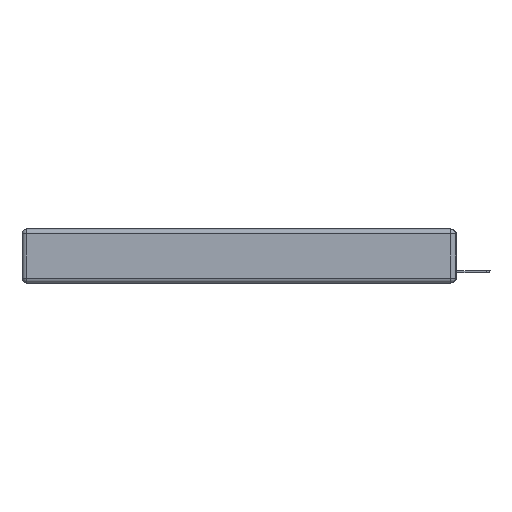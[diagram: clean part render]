
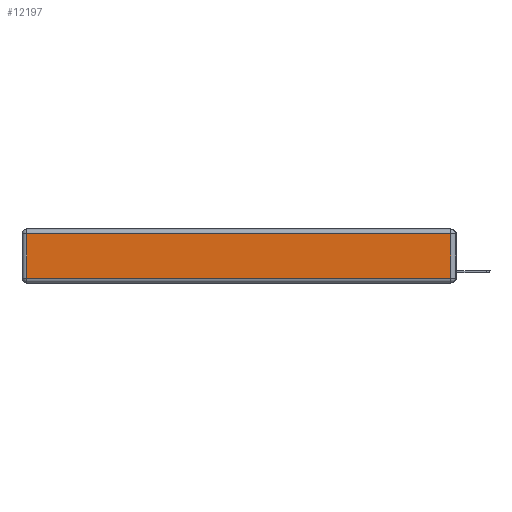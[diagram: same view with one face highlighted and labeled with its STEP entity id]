
A CAD part, left-side view. The second image highlights one B-rep face of the part: STEP entity #12197.
In plain terms, the highlighted planar face has unit normal (-1, 0, 0).
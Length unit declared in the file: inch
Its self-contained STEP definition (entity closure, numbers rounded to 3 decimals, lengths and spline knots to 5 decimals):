
#1809 = AXIS2_PLACEMENT_3D ( 'NONE', #8646, #13525, #8936 ) ;
#2322 = CARTESIAN_POINT ( 'NONE',  ( 0., 0.03, -0.03 ) ) ;
#3725 = EDGE_CURVE ( 'NONE', #6217, #6629, #13853, .T. ) ;
#4419 = ORIENTED_EDGE ( 'NONE', *, *, #15824, .T. ) ;
#4536 = LINE ( 'NONE', #9235, #6363 ) ;
#5135 = PLANE ( 'NONE',  #1809 ) ;
#6217 = VERTEX_POINT ( 'NONE', #11369 ) ;
#6363 = VECTOR ( 'NONE', #21067, 39.37008 ) ;
#6536 = LINE ( 'NONE', #21518, #16589 ) ;
#6629 = VERTEX_POINT ( 'NONE', #2322 ) ;
#7221 = CARTESIAN_POINT ( 'NONE',  ( 0., 2.72, -0.343 ) ) ;
#7976 = DIRECTION ( 'NONE',  ( 0., 0., 1. ) ) ;
#8363 = VERTEX_POINT ( 'NONE', #20079 ) ;
#8646 = CARTESIAN_POINT ( 'NONE',  ( 0., 0., -0.343 ) ) ;
#8843 = DIRECTION ( 'NONE',  ( 0., 0., -1. ) ) ;
#8936 = DIRECTION ( 'NONE',  ( 0., 0., 1. ) ) ;
#9235 = CARTESIAN_POINT ( 'NONE',  ( 0., 2.75, -0.03 ) ) ;
#9616 = VECTOR ( 'NONE', #8843, 39.37008 ) ;
#9675 = EDGE_CURVE ( 'NONE', #6629, #8363, #4536, .T. ) ;
#10180 = EDGE_CURVE ( 'NONE', #8363, #13931, #19923, .T. ) ;
#11369 = CARTESIAN_POINT ( 'NONE',  ( 0., 0.03, -0.313 ) ) ;
#12197 = ADVANCED_FACE ( 'NONE', ( #12681 ), #5135, .T. ) ;
#12681 = FACE_OUTER_BOUND ( 'NONE', #14094, .T. ) ;
#13000 = CARTESIAN_POINT ( 'NONE',  ( 0., 2.72, -0.313 ) ) ;
#13525 = DIRECTION ( 'NONE',  ( -1., 0., 0. ) ) ;
#13853 = LINE ( 'NONE', #18116, #18639 ) ;
#13931 = VERTEX_POINT ( 'NONE', #13000 ) ;
#14094 = EDGE_LOOP ( 'NONE', ( #4419, #20969, #14578, #15767 ) ) ;
#14420 = DIRECTION ( 'NONE',  ( 0., -1., 0. ) ) ;
#14578 = ORIENTED_EDGE ( 'NONE', *, *, #9675, .T. ) ;
#15767 = ORIENTED_EDGE ( 'NONE', *, *, #10180, .T. ) ;
#15824 = EDGE_CURVE ( 'NONE', #13931, #6217, #6536, .T. ) ;
#16589 = VECTOR ( 'NONE', #14420, 39.37008 ) ;
#18116 = CARTESIAN_POINT ( 'NONE',  ( 0., 0.03, -0.343 ) ) ;
#18639 = VECTOR ( 'NONE', #7976, 39.37008 ) ;
#19923 = LINE ( 'NONE', #7221, #9616 ) ;
#20079 = CARTESIAN_POINT ( 'NONE',  ( 0., 2.72, -0.03 ) ) ;
#20969 = ORIENTED_EDGE ( 'NONE', *, *, #3725, .T. ) ;
#21067 = DIRECTION ( 'NONE',  ( 0., 1., 0. ) ) ;
#21518 = CARTESIAN_POINT ( 'NONE',  ( 0., 0., -0.313 ) ) ;
